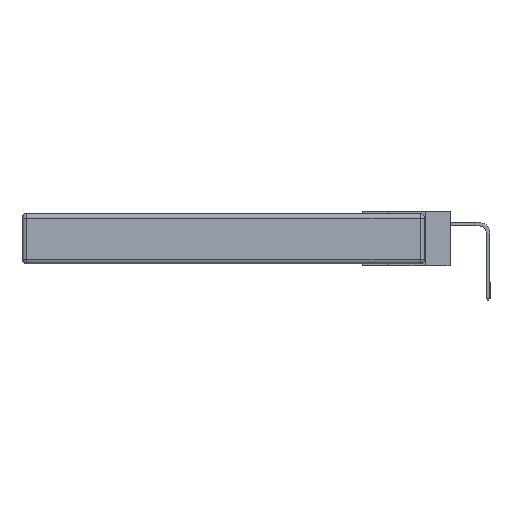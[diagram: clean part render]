
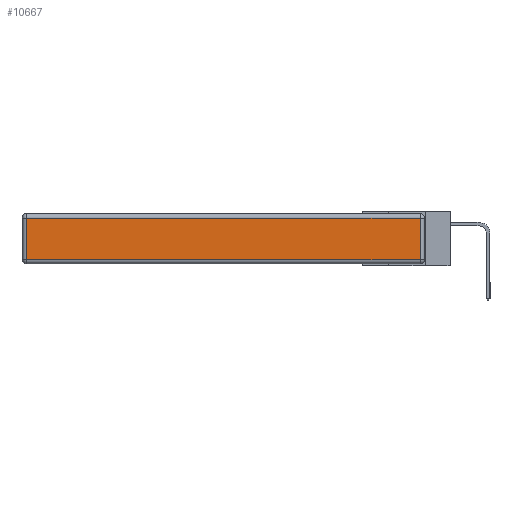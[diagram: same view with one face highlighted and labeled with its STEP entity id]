
A CAD part, left-side view. The second image highlights one B-rep face of the part: STEP entity #10667.
In plain terms, the highlighted planar face has unit normal (-1, 0, 0).
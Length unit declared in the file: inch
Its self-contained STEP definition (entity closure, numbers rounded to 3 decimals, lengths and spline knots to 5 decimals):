
#102 = LINE ( 'NONE', #11076, #853 ) ;
#853 = VECTOR ( 'NONE', #3182, 39.37008 ) ;
#1175 = LINE ( 'NONE', #6766, #8138 ) ;
#1776 = EDGE_CURVE ( 'NONE', #2146, #10390, #2608, .T. ) ;
#2009 = FACE_OUTER_BOUND ( 'NONE', #9010, .T. ) ;
#2146 = VERTEX_POINT ( 'NONE', #2570 ) ;
#2570 = CARTESIAN_POINT ( 'NONE',  ( 0., 2.72, -0.313 ) ) ;
#2608 = LINE ( 'NONE', #7436, #5834 ) ;
#2741 = DIRECTION ( 'NONE',  ( 0., 0., 1. ) ) ;
#3182 = DIRECTION ( 'NONE',  ( 0., 0., 1. ) ) ;
#3573 = AXIS2_PLACEMENT_3D ( 'NONE', #8567, #4703, #2741 ) ;
#3608 = CARTESIAN_POINT ( 'NONE',  ( 0., 2.72, -0.03 ) ) ;
#4056 = VECTOR ( 'NONE', #5393, 39.37008 ) ;
#4164 = VERTEX_POINT ( 'NONE', #9825 ) ;
#4289 = EDGE_CURVE ( 'NONE', #10390, #4164, #102, .T. ) ;
#4596 = DIRECTION ( 'NONE',  ( 0., -1., 0. ) ) ;
#4703 = DIRECTION ( 'NONE',  ( -1., 0., 0. ) ) ;
#4896 = DIRECTION ( 'NONE',  ( 0., 0., -1. ) ) ;
#5393 = DIRECTION ( 'NONE',  ( 0., 1., 0. ) ) ;
#5798 = ORIENTED_EDGE ( 'NONE', *, *, #7066, .T. ) ;
#5834 = VECTOR ( 'NONE', #4596, 39.37008 ) ;
#6663 = PLANE ( 'NONE',  #3573 ) ;
#6766 = CARTESIAN_POINT ( 'NONE',  ( 0., 2.72, -0.343 ) ) ;
#6849 = LINE ( 'NONE', #9294, #4056 ) ;
#7066 = EDGE_CURVE ( 'NONE', #10094, #2146, #1175, .T. ) ;
#7090 = ORIENTED_EDGE ( 'NONE', *, *, #1776, .T. ) ;
#7436 = CARTESIAN_POINT ( 'NONE',  ( 0., 0., -0.313 ) ) ;
#7991 = CARTESIAN_POINT ( 'NONE',  ( 0., 0.03, -0.313 ) ) ;
#8138 = VECTOR ( 'NONE', #4896, 39.37008 ) ;
#8309 = EDGE_CURVE ( 'NONE', #4164, #10094, #6849, .T. ) ;
#8567 = CARTESIAN_POINT ( 'NONE',  ( 0., 0., -0.343 ) ) ;
#8934 = ORIENTED_EDGE ( 'NONE', *, *, #8309, .T. ) ;
#9010 = EDGE_LOOP ( 'NONE', ( #7090, #9556, #8934, #5798 ) ) ;
#9294 = CARTESIAN_POINT ( 'NONE',  ( 0., 2.75, -0.03 ) ) ;
#9556 = ORIENTED_EDGE ( 'NONE', *, *, #4289, .T. ) ;
#9825 = CARTESIAN_POINT ( 'NONE',  ( 0., 0.03, -0.03 ) ) ;
#10094 = VERTEX_POINT ( 'NONE', #3608 ) ;
#10390 = VERTEX_POINT ( 'NONE', #7991 ) ;
#10667 = ADVANCED_FACE ( 'NONE', ( #2009 ), #6663, .T. ) ;
#11076 = CARTESIAN_POINT ( 'NONE',  ( 0., 0.03, -0.343 ) ) ;
